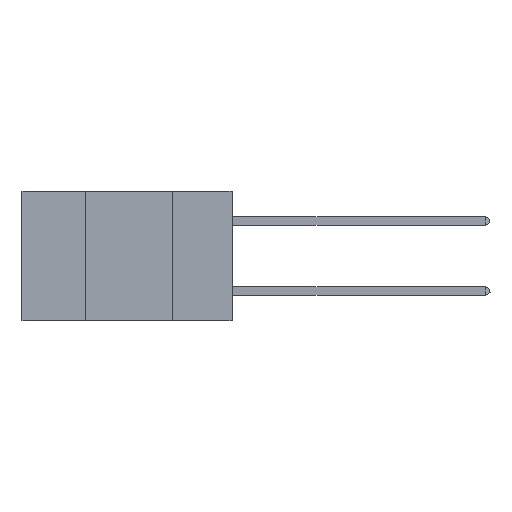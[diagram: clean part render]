
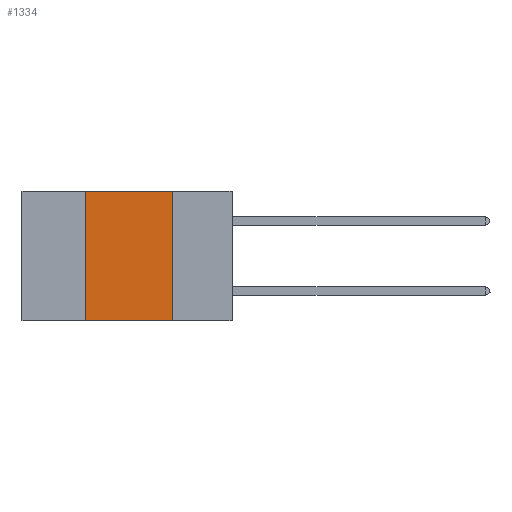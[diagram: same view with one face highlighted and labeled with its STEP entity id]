
A CAD part, left-side view. The second image highlights one B-rep face of the part: STEP entity #1334.
In plain terms, the highlighted planar face has unit normal (-1, 0, 0).
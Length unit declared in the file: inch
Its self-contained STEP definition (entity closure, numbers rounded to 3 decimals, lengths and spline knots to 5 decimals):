
#450 = VECTOR ( 'NONE', #7923, 39.37008 ) ;
#878 = CARTESIAN_POINT ( 'NONE',  ( 0., 0.6, 0. ) ) ;
#1232 = CARTESIAN_POINT ( 'NONE',  ( 0., 0.42, 0. ) ) ;
#1334 = ADVANCED_FACE ( 'NONE', ( #2997 ), #1752, .F. ) ;
#1352 = VERTEX_POINT ( 'NONE', #1874 ) ;
#1570 = EDGE_CURVE ( 'NONE', #3461, #4079, #1900, .T. ) ;
#1571 = VECTOR ( 'NONE', #5876, 39.37008 ) ;
#1752 = PLANE ( 'NONE',  #6319 ) ;
#1874 = CARTESIAN_POINT ( 'NONE',  ( 0., 0.17, 0. ) ) ;
#1900 = LINE ( 'NONE', #2835, #450 ) ;
#2353 = ORIENTED_EDGE ( 'NONE', *, *, #2813, .F. ) ;
#2397 = ORIENTED_EDGE ( 'NONE', *, *, #6946, .F. ) ;
#2474 = VERTEX_POINT ( 'NONE', #1232 ) ;
#2640 = DIRECTION ( 'NONE',  ( 1., 0., 0. ) ) ;
#2813 = EDGE_CURVE ( 'NONE', #3461, #2474, #7620, .T. ) ;
#2835 = CARTESIAN_POINT ( 'NONE',  ( 0., 0.6, -0.37 ) ) ;
#2997 = FACE_OUTER_BOUND ( 'NONE', #4907, .T. ) ;
#3452 = VECTOR ( 'NONE', #6708, 39.37008 ) ;
#3461 = VERTEX_POINT ( 'NONE', #7031 ) ;
#4079 = VERTEX_POINT ( 'NONE', #7157 ) ;
#4142 = ORIENTED_EDGE ( 'NONE', *, *, #7044, .F. ) ;
#4334 = CARTESIAN_POINT ( 'NONE',  ( 0., 0.42, 0. ) ) ;
#4907 = EDGE_LOOP ( 'NONE', ( #4142, #2397, #2353, #9907 ) ) ;
#5239 = DIRECTION ( 'NONE',  ( 0., 0., -1. ) ) ;
#5756 = CARTESIAN_POINT ( 'NONE',  ( 0., 0.6, 0. ) ) ;
#5876 = DIRECTION ( 'NONE',  ( 0., 0., -1. ) ) ;
#6158 = DIRECTION ( 'NONE',  ( 0., 0., 1. ) ) ;
#6319 = AXIS2_PLACEMENT_3D ( 'NONE', #878, #2640, #5239 ) ;
#6708 = DIRECTION ( 'NONE',  ( 0., -1., 0. ) ) ;
#6946 = EDGE_CURVE ( 'NONE', #2474, #1352, #7520, .T. ) ;
#7031 = CARTESIAN_POINT ( 'NONE',  ( 0., 0.42, -0.37 ) ) ;
#7044 = EDGE_CURVE ( 'NONE', #1352, #4079, #10651, .T. ) ;
#7157 = CARTESIAN_POINT ( 'NONE',  ( 0., 0.17, -0.37 ) ) ;
#7520 = LINE ( 'NONE', #5756, #3452 ) ;
#7620 = LINE ( 'NONE', #4334, #9235 ) ;
#7923 = DIRECTION ( 'NONE',  ( 0., -1., 0. ) ) ;
#9235 = VECTOR ( 'NONE', #6158, 39.37008 ) ;
#9399 = CARTESIAN_POINT ( 'NONE',  ( 0., 0.17, 0. ) ) ;
#9907 = ORIENTED_EDGE ( 'NONE', *, *, #1570, .T. ) ;
#10651 = LINE ( 'NONE', #9399, #1571 ) ;
